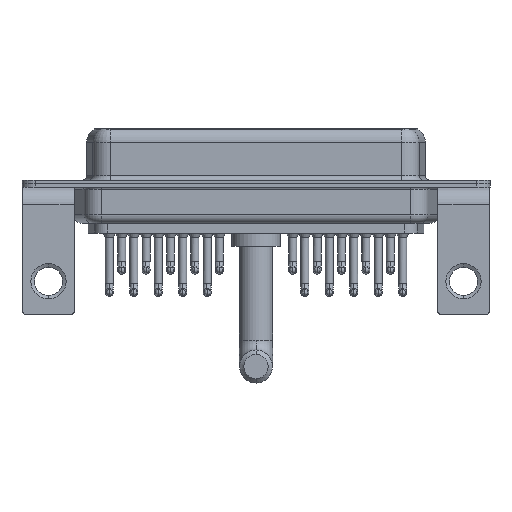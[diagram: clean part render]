
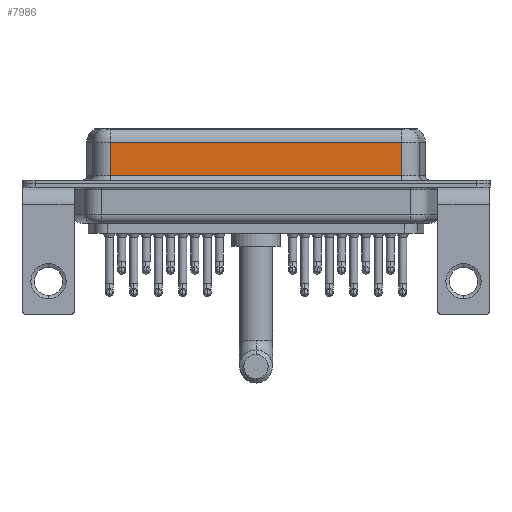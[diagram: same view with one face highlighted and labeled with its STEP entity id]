
A CAD part, front view. The second image highlights one B-rep face of the part: STEP entity #7986.
In plain terms, the highlighted planar face has unit normal (0, -1, 0).
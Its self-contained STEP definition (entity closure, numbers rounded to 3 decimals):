
#2018 = DIRECTION ( 'NONE',  ( -1., 0., 0. ) ) ;
#2221 = VECTOR ( 'NONE', #10686, 1000. ) ;
#3603 = EDGE_CURVE ( 'NONE', #6801, #13579, #14459, .T. ) ;
#5381 = CARTESIAN_POINT ( 'NONE',  ( 7.013, -3.95, 0.9 ) ) ;
#5566 = LINE ( 'NONE', #20023, #8223 ) ;
#6255 = VECTOR ( 'NONE', #18790, 1000. ) ;
#6801 = VERTEX_POINT ( 'NONE', #10551 ) ;
#7986 = ADVANCED_FACE ( 'NONE', ( #11396 ), #14939, .F. ) ;
#8223 = VECTOR ( 'NONE', #11009, 1000. ) ;
#8385 = EDGE_LOOP ( 'NONE', ( #9623, #21910, #23387, #14624 ) ) ;
#9272 = CARTESIAN_POINT ( 'NONE',  ( 7.013, -3.95, 6.4 ) ) ;
#9623 = ORIENTED_EDGE ( 'NONE', *, *, #3603, .F. ) ;
#10446 = VERTEX_POINT ( 'NONE', #5381 ) ;
#10551 = CARTESIAN_POINT ( 'NONE',  ( 40.037, -3.95, 4.65 ) ) ;
#10593 = EDGE_CURVE ( 'NONE', #20709, #10446, #13198, .T. ) ;
#10686 = DIRECTION ( 'NONE',  ( 0., 0., -1. ) ) ;
#11009 = DIRECTION ( 'NONE',  ( 1., 0., 0. ) ) ;
#11396 = FACE_OUTER_BOUND ( 'NONE', #8385, .T. ) ;
#11629 = DIRECTION ( 'NONE',  ( 0., 1., 0. ) ) ;
#12104 = EDGE_CURVE ( 'NONE', #10446, #13579, #5566, .T. ) ;
#13002 = AXIS2_PLACEMENT_3D ( 'NONE', #22061, #11629, #20517 ) ;
#13198 = LINE ( 'NONE', #9272, #6255 ) ;
#13482 = EDGE_CURVE ( 'NONE', #6801, #20709, #14423, .T. ) ;
#13579 = VERTEX_POINT ( 'NONE', #18369 ) ;
#14423 = LINE ( 'NONE', #21680, #23374 ) ;
#14459 = LINE ( 'NONE', #19820, #2221 ) ;
#14624 = ORIENTED_EDGE ( 'NONE', *, *, #12104, .T. ) ;
#14939 = PLANE ( 'NONE',  #13002 ) ;
#15451 = CARTESIAN_POINT ( 'NONE',  ( 7.013, -3.95, 4.65 ) ) ;
#18369 = CARTESIAN_POINT ( 'NONE',  ( 40.037, -3.95, 0.9 ) ) ;
#18790 = DIRECTION ( 'NONE',  ( 0., 0., -1. ) ) ;
#19820 = CARTESIAN_POINT ( 'NONE',  ( 40.037, -3.95, 6.4 ) ) ;
#20023 = CARTESIAN_POINT ( 'NONE',  ( 40.037, -3.95, 0.9 ) ) ;
#20517 = DIRECTION ( 'NONE',  ( 0., 0., 1. ) ) ;
#20709 = VERTEX_POINT ( 'NONE', #15451 ) ;
#21680 = CARTESIAN_POINT ( 'NONE',  ( 40.037, -3.95, 4.65 ) ) ;
#21910 = ORIENTED_EDGE ( 'NONE', *, *, #13482, .T. ) ;
#22061 = CARTESIAN_POINT ( 'NONE',  ( 40.037, -3.95, 6.4 ) ) ;
#23374 = VECTOR ( 'NONE', #2018, 1000. ) ;
#23387 = ORIENTED_EDGE ( 'NONE', *, *, #10593, .T. ) ;
